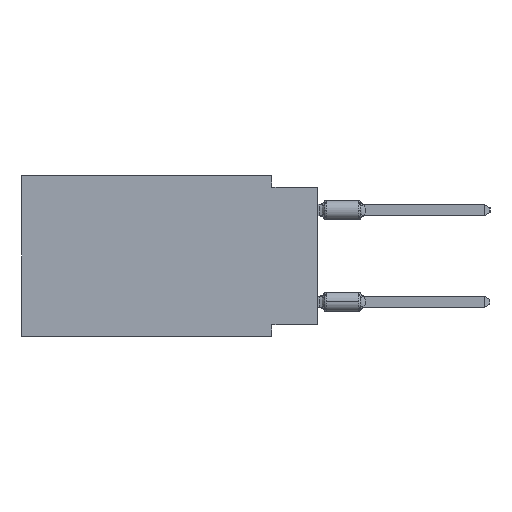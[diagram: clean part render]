
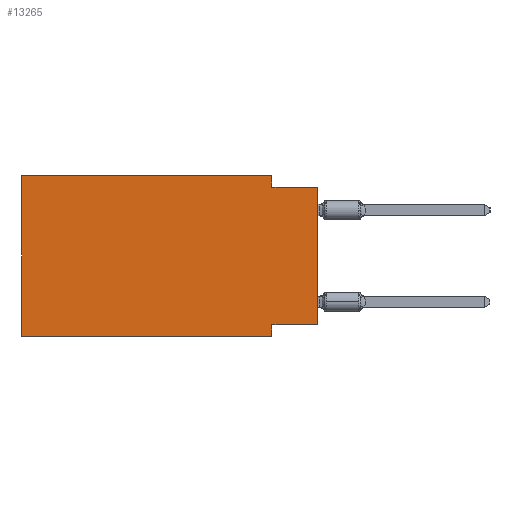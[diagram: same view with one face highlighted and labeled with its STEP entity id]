
A CAD part, left-side view. The second image highlights one B-rep face of the part: STEP entity #13265.
In plain terms, the highlighted planar face has unit normal (-1, 0, 0).
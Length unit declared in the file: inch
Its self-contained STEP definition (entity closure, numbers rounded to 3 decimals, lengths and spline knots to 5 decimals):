
#250 = VECTOR ( 'NONE', #10857, 39.37008 ) ;
#281 = CARTESIAN_POINT ( 'NONE',  ( 0., 0.1, -0.35 ) ) ;
#1295 = CARTESIAN_POINT ( 'NONE',  ( 0., 0.645, 0. ) ) ;
#2333 = FACE_OUTER_BOUND ( 'NONE', #13622, .T. ) ;
#2908 = CARTESIAN_POINT ( 'NONE',  ( 0., 0.645, -0.35 ) ) ;
#3362 = ORIENTED_EDGE ( 'NONE', *, *, #4404, .F. ) ;
#3628 = LINE ( 'NONE', #8409, #17043 ) ;
#4404 = EDGE_CURVE ( 'NONE', #30665, #9648, #3628, .T. ) ;
#5751 = EDGE_CURVE ( 'NONE', #13566, #31074, #13599, .T. ) ;
#6015 = CARTESIAN_POINT ( 'NONE',  ( 0., 0.1, -0.025 ) ) ;
#6287 = VERTEX_POINT ( 'NONE', #17315 ) ;
#6522 = CARTESIAN_POINT ( 'NONE',  ( 0., 0.1, -0.35 ) ) ;
#6791 = VERTEX_POINT ( 'NONE', #10496 ) ;
#7338 = VECTOR ( 'NONE', #12513, 39.37008 ) ;
#8003 = LINE ( 'NONE', #2908, #27784 ) ;
#8316 = VECTOR ( 'NONE', #24017, 39.37008 ) ;
#8345 = ORIENTED_EDGE ( 'NONE', *, *, #12295, .T. ) ;
#8409 = CARTESIAN_POINT ( 'NONE',  ( 0., 0., -0.325 ) ) ;
#8411 = EDGE_CURVE ( 'NONE', #9648, #31697, #20068, .T. ) ;
#8756 = EDGE_CURVE ( 'NONE', #6287, #13566, #21391, .T. ) ;
#8917 = CARTESIAN_POINT ( 'NONE',  ( 0., 0., 0. ) ) ;
#8979 = DIRECTION ( 'NONE',  ( 0., -1., 0. ) ) ;
#9464 = CARTESIAN_POINT ( 'NONE',  ( 0., 0.645, -0.35 ) ) ;
#9648 = VERTEX_POINT ( 'NONE', #15429 ) ;
#10183 = VECTOR ( 'NONE', #11696, 39.37008 ) ;
#10496 = CARTESIAN_POINT ( 'NONE',  ( 0., 0.645, 0. ) ) ;
#10857 = DIRECTION ( 'NONE',  ( 0., -1., 0. ) ) ;
#11696 = DIRECTION ( 'NONE',  ( 0., 0., 1. ) ) ;
#11990 = CARTESIAN_POINT ( 'NONE',  ( 0., 0., -0.325 ) ) ;
#12295 = EDGE_CURVE ( 'NONE', #30665, #31074, #23590, .T. ) ;
#12331 = DIRECTION ( 'NONE',  ( 0., 0., -1. ) ) ;
#12513 = DIRECTION ( 'NONE',  ( 0., 0., 1. ) ) ;
#13265 = ADVANCED_FACE ( 'NONE', ( #2333 ), #15029, .F. ) ;
#13566 = VERTEX_POINT ( 'NONE', #6015 ) ;
#13599 = LINE ( 'NONE', #31063, #15528 ) ;
#13622 = EDGE_LOOP ( 'NONE', ( #8345, #18003, #25937, #32492, #32486, #24778, #24110, #3362 ) ) ;
#14090 = VECTOR ( 'NONE', #12331, 39.37008 ) ;
#15029 = PLANE ( 'NONE',  #20754 ) ;
#15064 = VERTEX_POINT ( 'NONE', #9464 ) ;
#15429 = CARTESIAN_POINT ( 'NONE',  ( 0., 0.1, -0.325 ) ) ;
#15528 = VECTOR ( 'NONE', #8979, 39.37008 ) ;
#17043 = VECTOR ( 'NONE', #26373, 39.37008 ) ;
#17315 = CARTESIAN_POINT ( 'NONE',  ( 0., 0.1, 0. ) ) ;
#18003 = ORIENTED_EDGE ( 'NONE', *, *, #5751, .F. ) ;
#18050 = DIRECTION ( 'NONE',  ( 0., -1., 0. ) ) ;
#20068 = LINE ( 'NONE', #281, #14090 ) ;
#20078 = CARTESIAN_POINT ( 'NONE',  ( 0., 0.645, 0. ) ) ;
#20754 = AXIS2_PLACEMENT_3D ( 'NONE', #32170, #27396, #27718 ) ;
#21391 = LINE ( 'NONE', #28959, #8316 ) ;
#23590 = LINE ( 'NONE', #8917, #10183 ) ;
#23865 = LINE ( 'NONE', #1295, #250 ) ;
#24017 = DIRECTION ( 'NONE',  ( 0., 0., -1. ) ) ;
#24110 = ORIENTED_EDGE ( 'NONE', *, *, #8411, .F. ) ;
#24778 = ORIENTED_EDGE ( 'NONE', *, *, #28401, .T. ) ;
#25325 = EDGE_CURVE ( 'NONE', #6791, #6287, #23865, .T. ) ;
#25937 = ORIENTED_EDGE ( 'NONE', *, *, #8756, .F. ) ;
#26373 = DIRECTION ( 'NONE',  ( 0., 1., 0. ) ) ;
#27396 = DIRECTION ( 'NONE',  ( 1., 0., 0. ) ) ;
#27718 = DIRECTION ( 'NONE',  ( 0., 0., -1. ) ) ;
#27784 = VECTOR ( 'NONE', #18050, 39.37008 ) ;
#28153 = LINE ( 'NONE', #20078, #7338 ) ;
#28401 = EDGE_CURVE ( 'NONE', #15064, #31697, #8003, .T. ) ;
#28959 = CARTESIAN_POINT ( 'NONE',  ( 0., 0.1, 0. ) ) ;
#29640 = CARTESIAN_POINT ( 'NONE',  ( 0., 0., -0.025 ) ) ;
#30665 = VERTEX_POINT ( 'NONE', #11990 ) ;
#31063 = CARTESIAN_POINT ( 'NONE',  ( 0., 0., -0.025 ) ) ;
#31074 = VERTEX_POINT ( 'NONE', #29640 ) ;
#31554 = EDGE_CURVE ( 'NONE', #15064, #6791, #28153, .T. ) ;
#31697 = VERTEX_POINT ( 'NONE', #6522 ) ;
#32170 = CARTESIAN_POINT ( 'NONE',  ( 0., 0.645, 0. ) ) ;
#32486 = ORIENTED_EDGE ( 'NONE', *, *, #31554, .F. ) ;
#32492 = ORIENTED_EDGE ( 'NONE', *, *, #25325, .F. ) ;
